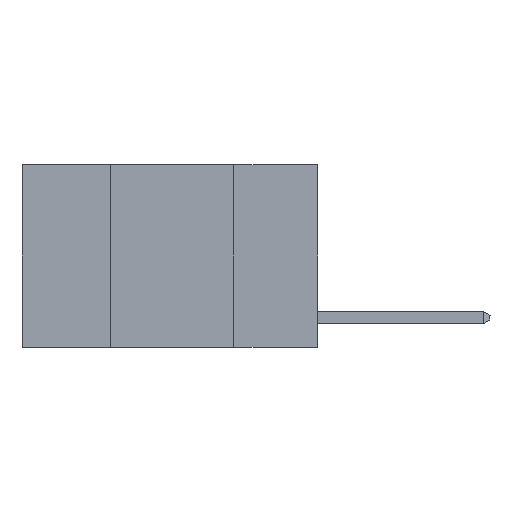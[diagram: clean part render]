
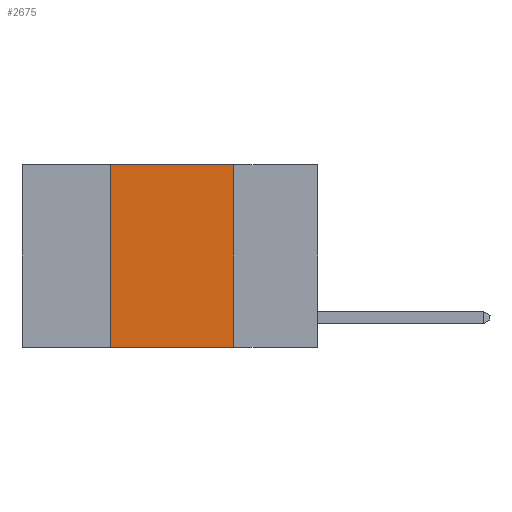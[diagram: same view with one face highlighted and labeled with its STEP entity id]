
A CAD part, left-side view. The second image highlights one B-rep face of the part: STEP entity #2675.
In plain terms, the highlighted planar face has unit normal (-1, 0, 0).
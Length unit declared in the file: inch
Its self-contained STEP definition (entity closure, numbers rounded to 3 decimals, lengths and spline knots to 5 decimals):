
#442 = CARTESIAN_POINT ( 'NONE',  ( 0., 0.42, 0. ) ) ;
#766 = CARTESIAN_POINT ( 'NONE',  ( 0., 0.17, 0. ) ) ;
#828 = DIRECTION ( 'NONE',  ( 0., 0., -1. ) ) ;
#2081 = CARTESIAN_POINT ( 'NONE',  ( 0., 0.6, 0. ) ) ;
#2407 = DIRECTION ( 'NONE',  ( 0., 0., 1. ) ) ;
#2675 = ADVANCED_FACE ( 'NONE', ( #8226 ), #13367, .F. ) ;
#2994 = ORIENTED_EDGE ( 'NONE', *, *, #9364, .F. ) ;
#3391 = VERTEX_POINT ( 'NONE', #9925 ) ;
#3590 = ORIENTED_EDGE ( 'NONE', *, *, #7058, .T. ) ;
#3646 = VECTOR ( 'NONE', #2407, 39.37008 ) ;
#4689 = EDGE_CURVE ( 'NONE', #6423, #17680, #13710, .T. ) ;
#5912 = DIRECTION ( 'NONE',  ( 0., 0., -1. ) ) ;
#6036 = EDGE_CURVE ( 'NONE', #17680, #3391, #7494, .T. ) ;
#6423 = VERTEX_POINT ( 'NONE', #9458 ) ;
#7058 = EDGE_CURVE ( 'NONE', #14833, #3391, #15203, .T. ) ;
#7494 = LINE ( 'NONE', #23264, #16903 ) ;
#8226 = FACE_OUTER_BOUND ( 'NONE', #11704, .T. ) ;
#9364 = EDGE_CURVE ( 'NONE', #14833, #6423, #18044, .T. ) ;
#9458 = CARTESIAN_POINT ( 'NONE',  ( 0., 0.42, 0. ) ) ;
#9925 = CARTESIAN_POINT ( 'NONE',  ( 0., 0.17, -0.37 ) ) ;
#10222 = VECTOR ( 'NONE', #19230, 39.37008 ) ;
#11704 = EDGE_LOOP ( 'NONE', ( #20600, #11820, #2994, #3590 ) ) ;
#11820 = ORIENTED_EDGE ( 'NONE', *, *, #4689, .F. ) ;
#13367 = PLANE ( 'NONE',  #18518 ) ;
#13710 = LINE ( 'NONE', #21359, #17541 ) ;
#13920 = DIRECTION ( 'NONE',  ( 0., -1., 0. ) ) ;
#14833 = VERTEX_POINT ( 'NONE', #19026 ) ;
#15203 = LINE ( 'NONE', #22834, #10222 ) ;
#16903 = VECTOR ( 'NONE', #828, 39.37008 ) ;
#17169 = DIRECTION ( 'NONE',  ( 1., 0., 0. ) ) ;
#17541 = VECTOR ( 'NONE', #13920, 39.37008 ) ;
#17680 = VERTEX_POINT ( 'NONE', #766 ) ;
#18044 = LINE ( 'NONE', #442, #3646 ) ;
#18518 = AXIS2_PLACEMENT_3D ( 'NONE', #2081, #17169, #5912 ) ;
#19026 = CARTESIAN_POINT ( 'NONE',  ( 0., 0.42, -0.37 ) ) ;
#19230 = DIRECTION ( 'NONE',  ( 0., -1., 0. ) ) ;
#20600 = ORIENTED_EDGE ( 'NONE', *, *, #6036, .F. ) ;
#21359 = CARTESIAN_POINT ( 'NONE',  ( 0., 0.6, 0. ) ) ;
#22834 = CARTESIAN_POINT ( 'NONE',  ( 0., 0.6, -0.37 ) ) ;
#23264 = CARTESIAN_POINT ( 'NONE',  ( 0., 0.17, 0. ) ) ;
